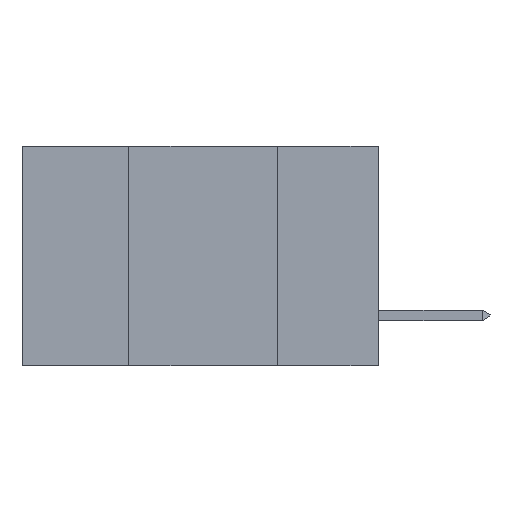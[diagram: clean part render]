
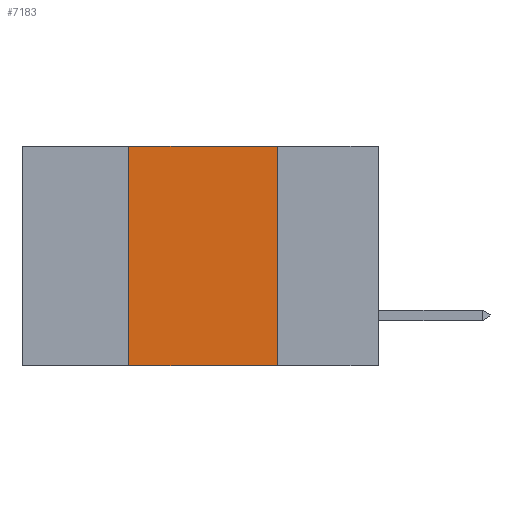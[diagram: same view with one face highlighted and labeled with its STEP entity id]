
A CAD part, left-side view. The second image highlights one B-rep face of the part: STEP entity #7183.
In plain terms, the highlighted planar face has unit normal (-1, 0, 0).
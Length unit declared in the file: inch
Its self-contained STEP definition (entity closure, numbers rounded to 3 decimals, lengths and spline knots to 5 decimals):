
#89 = LINE ( 'NONE', #938, #3901 ) ;
#155 = ORIENTED_EDGE ( 'NONE', *, *, #7824, .F. ) ;
#277 = EDGE_CURVE ( 'NONE', #1423, #2435, #5201, .T. ) ;
#604 = ORIENTED_EDGE ( 'NONE', *, *, #4216, .T. ) ;
#802 = DIRECTION ( 'NONE',  ( 0., 0., 1. ) ) ;
#938 = CARTESIAN_POINT ( 'NONE',  ( 0., 0.6, -0.37 ) ) ;
#992 = DIRECTION ( 'NONE',  ( 1., 0., 0. ) ) ;
#1067 = VERTEX_POINT ( 'NONE', #5110 ) ;
#1423 = VERTEX_POINT ( 'NONE', #2979 ) ;
#1576 = ORIENTED_EDGE ( 'NONE', *, *, #277, .F. ) ;
#1839 = EDGE_LOOP ( 'NONE', ( #8536, #1576, #155, #604 ) ) ;
#1896 = VECTOR ( 'NONE', #2783, 39.37008 ) ;
#2435 = VERTEX_POINT ( 'NONE', #9006 ) ;
#2645 = DIRECTION ( 'NONE',  ( 0., 0., -1. ) ) ;
#2783 = DIRECTION ( 'NONE',  ( 0., -1., 0. ) ) ;
#2979 = CARTESIAN_POINT ( 'NONE',  ( 0., 0.42, 0. ) ) ;
#3159 = AXIS2_PLACEMENT_3D ( 'NONE', #5182, #992, #2645 ) ;
#3224 = EDGE_CURVE ( 'NONE', #2435, #7899, #8081, .T. ) ;
#3401 = PLANE ( 'NONE',  #3159 ) ;
#3901 = VECTOR ( 'NONE', #5807, 39.37008 ) ;
#4139 = DIRECTION ( 'NONE',  ( 0., 0., -1. ) ) ;
#4216 = EDGE_CURVE ( 'NONE', #1067, #7899, #89, .T. ) ;
#5110 = CARTESIAN_POINT ( 'NONE',  ( 0., 0.42, -0.37 ) ) ;
#5182 = CARTESIAN_POINT ( 'NONE',  ( 0., 0.6, 0. ) ) ;
#5201 = LINE ( 'NONE', #10064, #1896 ) ;
#5807 = DIRECTION ( 'NONE',  ( 0., -1., 0. ) ) ;
#7183 = ADVANCED_FACE ( 'NONE', ( #9936 ), #3401, .F. ) ;
#7390 = CARTESIAN_POINT ( 'NONE',  ( 0., 0.17, -0.37 ) ) ;
#7496 = VECTOR ( 'NONE', #4139, 39.37008 ) ;
#7824 = EDGE_CURVE ( 'NONE', #1067, #1423, #9355, .T. ) ;
#7899 = VERTEX_POINT ( 'NONE', #10405 ) ;
#8081 = LINE ( 'NONE', #7390, #7496 ) ;
#8536 = ORIENTED_EDGE ( 'NONE', *, *, #3224, .F. ) ;
#8827 = CARTESIAN_POINT ( 'NONE',  ( 0., 0.42, -0.37 ) ) ;
#9006 = CARTESIAN_POINT ( 'NONE',  ( 0., 0.17, 0. ) ) ;
#9355 = LINE ( 'NONE', #8827, #10174 ) ;
#9936 = FACE_OUTER_BOUND ( 'NONE', #1839, .T. ) ;
#10064 = CARTESIAN_POINT ( 'NONE',  ( 0., 0.6, 0. ) ) ;
#10174 = VECTOR ( 'NONE', #802, 39.37008 ) ;
#10405 = CARTESIAN_POINT ( 'NONE',  ( 0., 0.17, -0.37 ) ) ;
